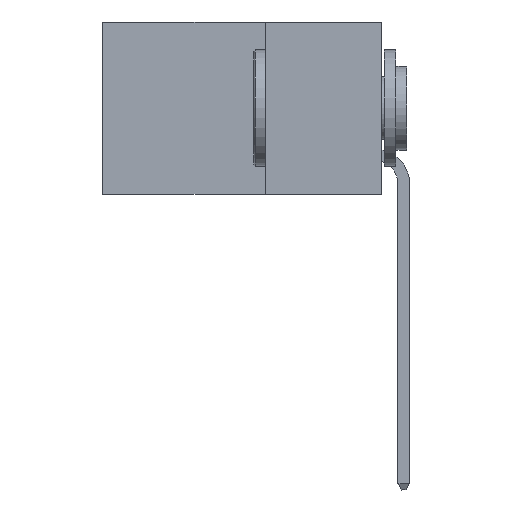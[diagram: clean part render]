
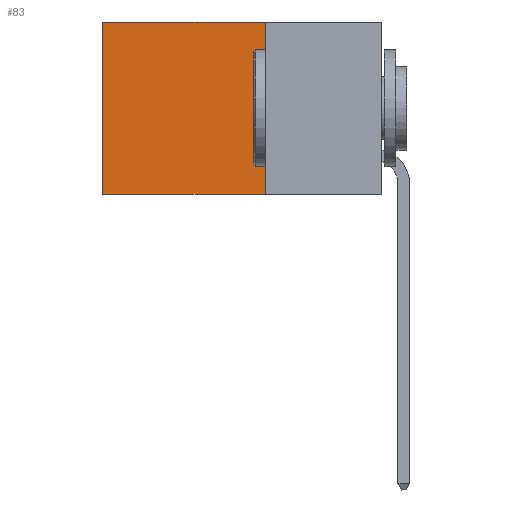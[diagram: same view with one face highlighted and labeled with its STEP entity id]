
A CAD part, left-side view. The second image highlights one B-rep face of the part: STEP entity #83.
In plain terms, the highlighted planar face has unit normal (-1, 0, 0).
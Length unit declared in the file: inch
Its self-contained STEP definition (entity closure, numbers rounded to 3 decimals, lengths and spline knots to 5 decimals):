
#83 = ADVANCED_FACE ( 'NONE', ( #8355 ), #6589, .F. ) ;
#374 = DIRECTION ( 'NONE',  ( 0., 0., -1. ) ) ;
#480 = ORIENTED_EDGE ( 'NONE', *, *, #11559, .T. ) ;
#637 = VECTOR ( 'NONE', #14074, 39.37008 ) ;
#1028 = VERTEX_POINT ( 'NONE', #4486 ) ;
#1166 = LINE ( 'NONE', #10942, #9289 ) ;
#4364 = EDGE_CURVE ( 'NONE', #6911, #20152, #7146, .T. ) ;
#4486 = CARTESIAN_POINT ( 'NONE',  ( 0.2875, 0.25, -0.37 ) ) ;
#4667 = ORIENTED_EDGE ( 'NONE', *, *, #6915, .F. ) ;
#4903 = CARTESIAN_POINT ( 'NONE',  ( 0.2875, 0.6, -0.37 ) ) ;
#6487 = CARTESIAN_POINT ( 'NONE',  ( 0.2875, 0.25, 0. ) ) ;
#6589 = PLANE ( 'NONE',  #19944 ) ;
#6697 = VECTOR ( 'NONE', #12855, 39.37008 ) ;
#6911 = VERTEX_POINT ( 'NONE', #14057 ) ;
#6915 = EDGE_CURVE ( 'NONE', #15875, #1028, #1166, .T. ) ;
#7146 = LINE ( 'NONE', #19432, #10903 ) ;
#7734 = DIRECTION ( 'NONE',  ( 1., 0., 0. ) ) ;
#7961 = EDGE_LOOP ( 'NONE', ( #18137, #8768, #4667, #480 ) ) ;
#8246 = LINE ( 'NONE', #12491, #637 ) ;
#8355 = FACE_OUTER_BOUND ( 'NONE', #7961, .T. ) ;
#8768 = ORIENTED_EDGE ( 'NONE', *, *, #9615, .F. ) ;
#9289 = VECTOR ( 'NONE', #18721, 39.37008 ) ;
#9615 = EDGE_CURVE ( 'NONE', #1028, #20152, #8246, .T. ) ;
#10903 = VECTOR ( 'NONE', #374, 39.37008 ) ;
#10942 = CARTESIAN_POINT ( 'NONE',  ( 0.2875, 0.25, 0. ) ) ;
#11374 = CARTESIAN_POINT ( 'NONE',  ( 0.2875, 0.25, 0. ) ) ;
#11559 = EDGE_CURVE ( 'NONE', #15875, #6911, #15153, .T. ) ;
#12491 = CARTESIAN_POINT ( 'NONE',  ( 0.2875, 0.25, -0.37 ) ) ;
#12855 = DIRECTION ( 'NONE',  ( 0., 1., 0. ) ) ;
#13278 = DIRECTION ( 'NONE',  ( 0., 0., -1. ) ) ;
#14057 = CARTESIAN_POINT ( 'NONE',  ( 0.2875, 0.6, 0. ) ) ;
#14074 = DIRECTION ( 'NONE',  ( 0., 1., 0. ) ) ;
#15153 = LINE ( 'NONE', #6487, #6697 ) ;
#15875 = VERTEX_POINT ( 'NONE', #11374 ) ;
#18106 = CARTESIAN_POINT ( 'NONE',  ( 0.2875, 0.25, 0. ) ) ;
#18137 = ORIENTED_EDGE ( 'NONE', *, *, #4364, .T. ) ;
#18721 = DIRECTION ( 'NONE',  ( 0., 0., -1. ) ) ;
#19432 = CARTESIAN_POINT ( 'NONE',  ( 0.2875, 0.6, 0. ) ) ;
#19944 = AXIS2_PLACEMENT_3D ( 'NONE', #18106, #7734, #13278 ) ;
#20152 = VERTEX_POINT ( 'NONE', #4903 ) ;
